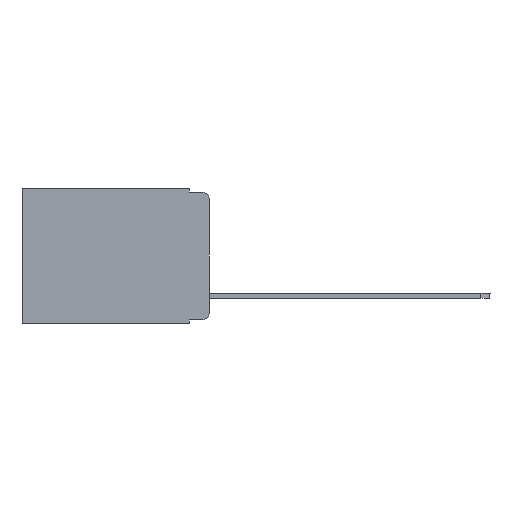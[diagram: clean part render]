
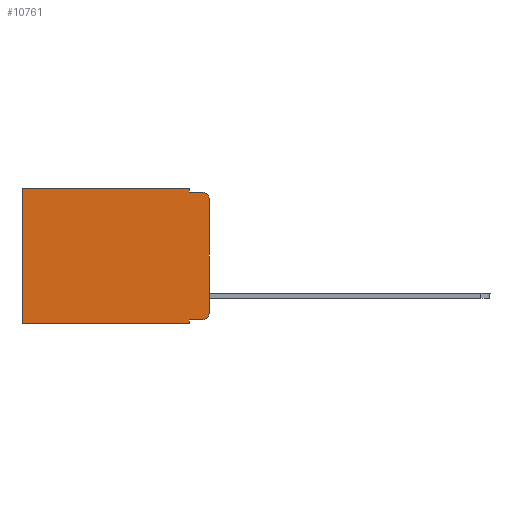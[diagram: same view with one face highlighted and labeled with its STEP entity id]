
A CAD part, left-side view. The second image highlights one B-rep face of the part: STEP entity #10761.
In plain terms, the highlighted planar face has unit normal (-1, 0, 0).
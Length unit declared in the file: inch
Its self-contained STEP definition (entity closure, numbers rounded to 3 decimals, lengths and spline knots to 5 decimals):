
#104 = DIRECTION ( 'NONE',  ( 0., 0., -1. ) ) ;
#379 = CARTESIAN_POINT ( 'NONE',  ( 0.298, 0., 0. ) ) ;
#597 = VERTEX_POINT ( 'NONE', #4473 ) ;
#640 = CARTESIAN_POINT ( 'NONE',  ( 0.298, 0.02, -0.313 ) ) ;
#835 = CARTESIAN_POINT ( 'NONE',  ( 0.298, 0., -0.03 ) ) ;
#939 = VECTOR ( 'NONE', #1279, 39.37008 ) ;
#1016 = DIRECTION ( 'NONE',  ( 0., 1., 0. ) ) ;
#1127 = CARTESIAN_POINT ( 'NONE',  ( 0.298, 0., 0. ) ) ;
#1279 = DIRECTION ( 'NONE',  ( 0., 0., -1. ) ) ;
#1379 = ORIENTED_EDGE ( 'NONE', *, *, #8041, .F. ) ;
#1394 = EDGE_CURVE ( 'NONE', #12761, #9390, #7551, .T. ) ;
#1556 = LINE ( 'NONE', #11075, #11870 ) ;
#1779 = DIRECTION ( 'NONE',  ( 0., 0., -1. ) ) ;
#1904 = CARTESIAN_POINT ( 'NONE',  ( 0.298, 0.473, 0. ) ) ;
#1970 = ORIENTED_EDGE ( 'NONE', *, *, #7031, .T. ) ;
#2284 = CARTESIAN_POINT ( 'NONE',  ( 0.298, 0.051, 0. ) ) ;
#2653 = ORIENTED_EDGE ( 'NONE', *, *, #8706, .F. ) ;
#2828 = EDGE_CURVE ( 'NONE', #11828, #2934, #9790, .T. ) ;
#2867 = CARTESIAN_POINT ( 'NONE',  ( 0.298, 0.051, 0. ) ) ;
#2908 = CARTESIAN_POINT ( 'NONE',  ( 0.298, 0.051, -0.01 ) ) ;
#2934 = VERTEX_POINT ( 'NONE', #5422 ) ;
#3256 = CARTESIAN_POINT ( 'NONE',  ( 0.298, 0.051, -0.01 ) ) ;
#3283 = DIRECTION ( 'NONE',  ( 0., -1., 0. ) ) ;
#3487 = CARTESIAN_POINT ( 'NONE',  ( 0.298, 0.051, 0. ) ) ;
#4473 = CARTESIAN_POINT ( 'NONE',  ( 0.298, 0.02, -0.01 ) ) ;
#4653 = EDGE_CURVE ( 'NONE', #12761, #10976, #11312, .T. ) ;
#4702 = LINE ( 'NONE', #8139, #12202 ) ;
#4816 = LINE ( 'NONE', #2908, #12621 ) ;
#5255 = EDGE_LOOP ( 'NONE', ( #2653, #1970, #1379, #7414, #7174, #10132, #11329, #8463, #7936, #9524 ) ) ;
#5422 = CARTESIAN_POINT ( 'NONE',  ( 0.298, 0.02, -0.333 ) ) ;
#5574 = VECTOR ( 'NONE', #3283, 39.37008 ) ;
#5678 = VECTOR ( 'NONE', #10902, 39.37008 ) ;
#5731 = CARTESIAN_POINT ( 'NONE',  ( 0.298, 0., -0.343 ) ) ;
#6042 = DIRECTION ( 'NONE',  ( 0., 0., -1. ) ) ;
#6424 = DIRECTION ( 'NONE',  ( 0., 0., -1. ) ) ;
#6512 = CARTESIAN_POINT ( 'NONE',  ( 0.298, 0.473, -0.343 ) ) ;
#6820 = CARTESIAN_POINT ( 'NONE',  ( 0.298, 0., -0.313 ) ) ;
#6952 = EDGE_CURVE ( 'NONE', #11828, #9382, #10150, .T. ) ;
#7031 = EDGE_CURVE ( 'NONE', #10312, #597, #9077, .T. ) ;
#7145 = AXIS2_PLACEMENT_3D ( 'NONE', #379, #7506, #6424 ) ;
#7174 = ORIENTED_EDGE ( 'NONE', *, *, #4653, .T. ) ;
#7414 = ORIENTED_EDGE ( 'NONE', *, *, #1394, .F. ) ;
#7506 = DIRECTION ( 'NONE',  ( 1., 0., 0. ) ) ;
#7551 = LINE ( 'NONE', #2867, #5678 ) ;
#7747 = LINE ( 'NONE', #5731, #8677 ) ;
#7787 = FACE_OUTER_BOUND ( 'NONE', #5255, .T. ) ;
#7895 = VECTOR ( 'NONE', #11208, 39.37008 ) ;
#7936 = ORIENTED_EDGE ( 'NONE', *, *, #2828, .T. ) ;
#8041 = EDGE_CURVE ( 'NONE', #9390, #597, #4816, .T. ) ;
#8139 = CARTESIAN_POINT ( 'NONE',  ( 0.298, 0., 0. ) ) ;
#8444 = DIRECTION ( 'NONE',  ( -1., 0., 0. ) ) ;
#8463 = ORIENTED_EDGE ( 'NONE', *, *, #6952, .F. ) ;
#8677 = VECTOR ( 'NONE', #1016, 39.37008 ) ;
#8706 = EDGE_CURVE ( 'NONE', #10312, #9095, #4702, .T. ) ;
#8773 = DIRECTION ( 'NONE',  ( -1., 0., 0. ) ) ;
#8800 = VERTEX_POINT ( 'NONE', #6512 ) ;
#8929 = EDGE_CURVE ( 'NONE', #2934, #9095, #10305, .T. ) ;
#9077 = CIRCLE ( 'NONE', #11943, 0.02 ) ;
#9095 = VERTEX_POINT ( 'NONE', #6820 ) ;
#9248 = CARTESIAN_POINT ( 'NONE',  ( 0.298, 0.051, -0.343 ) ) ;
#9296 = EDGE_CURVE ( 'NONE', #10976, #8800, #1556, .T. ) ;
#9382 = VERTEX_POINT ( 'NONE', #9248 ) ;
#9390 = VERTEX_POINT ( 'NONE', #3256 ) ;
#9422 = PLANE ( 'NONE',  #7145 ) ;
#9524 = ORIENTED_EDGE ( 'NONE', *, *, #8929, .T. ) ;
#9790 = LINE ( 'NONE', #12367, #5574 ) ;
#10132 = ORIENTED_EDGE ( 'NONE', *, *, #9296, .T. ) ;
#10150 = LINE ( 'NONE', #2284, #939 ) ;
#10305 = CIRCLE ( 'NONE', #11359, 0.02 ) ;
#10312 = VERTEX_POINT ( 'NONE', #835 ) ;
#10481 = CARTESIAN_POINT ( 'NONE',  ( 0.298, 0.02, -0.03 ) ) ;
#10761 = ADVANCED_FACE ( 'NONE', ( #7787 ), #9422, .F. ) ;
#10902 = DIRECTION ( 'NONE',  ( 0., 0., -1. ) ) ;
#10976 = VERTEX_POINT ( 'NONE', #1904 ) ;
#11068 = CARTESIAN_POINT ( 'NONE',  ( 0.298, 0.051, -0.333 ) ) ;
#11075 = CARTESIAN_POINT ( 'NONE',  ( 0.298, 0.473, 0. ) ) ;
#11208 = DIRECTION ( 'NONE',  ( 0., 1., 0. ) ) ;
#11312 = LINE ( 'NONE', #1127, #7895 ) ;
#11329 = ORIENTED_EDGE ( 'NONE', *, *, #12271, .F. ) ;
#11359 = AXIS2_PLACEMENT_3D ( 'NONE', #640, #8773, #1779 ) ;
#11828 = VERTEX_POINT ( 'NONE', #11068 ) ;
#11870 = VECTOR ( 'NONE', #104, 39.37008 ) ;
#11943 = AXIS2_PLACEMENT_3D ( 'NONE', #10481, #8444, #12581 ) ;
#11994 = DIRECTION ( 'NONE',  ( 0., -1., 0. ) ) ;
#12202 = VECTOR ( 'NONE', #6042, 39.37008 ) ;
#12271 = EDGE_CURVE ( 'NONE', #9382, #8800, #7747, .T. ) ;
#12367 = CARTESIAN_POINT ( 'NONE',  ( 0.298, 0.051, -0.333 ) ) ;
#12581 = DIRECTION ( 'NONE',  ( 0., 0., -1. ) ) ;
#12621 = VECTOR ( 'NONE', #11994, 39.37008 ) ;
#12761 = VERTEX_POINT ( 'NONE', #3487 ) ;
